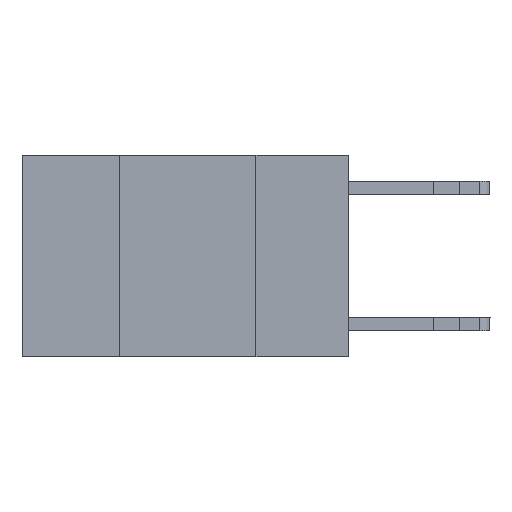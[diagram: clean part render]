
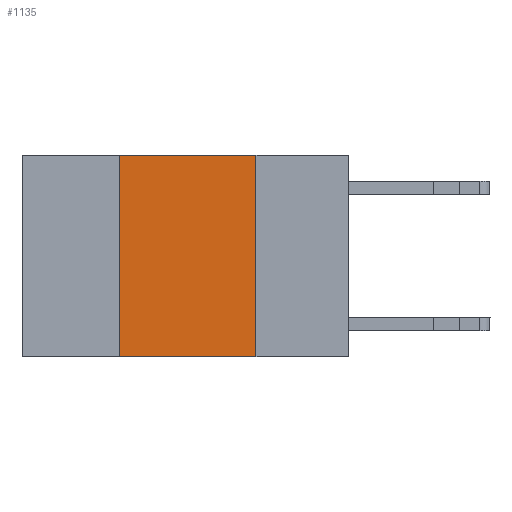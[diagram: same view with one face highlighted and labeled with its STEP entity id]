
A CAD part, left-side view. The second image highlights one B-rep face of the part: STEP entity #1135.
In plain terms, the highlighted planar face has unit normal (-1, 0, 0).
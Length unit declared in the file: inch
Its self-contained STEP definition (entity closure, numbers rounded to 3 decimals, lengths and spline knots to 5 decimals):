
#834 = DIRECTION ( 'NONE',  ( 0., 0., 1. ) ) ;
#880 = CARTESIAN_POINT ( 'NONE',  ( 0., 0.6, -0.37 ) ) ;
#1118 = CARTESIAN_POINT ( 'NONE',  ( 0., 0.17, -0.37 ) ) ;
#1135 = ADVANCED_FACE ( 'NONE', ( #6115 ), #10986, .F. ) ;
#1771 = ORIENTED_EDGE ( 'NONE', *, *, #2746, .T. ) ;
#1963 = ORIENTED_EDGE ( 'NONE', *, *, #4541, .F. ) ;
#2281 = ORIENTED_EDGE ( 'NONE', *, *, #16490, .F. ) ;
#2422 = LINE ( 'NONE', #9109, #12444 ) ;
#2746 = EDGE_CURVE ( 'NONE', #12424, #6067, #11753, .T. ) ;
#2831 = CARTESIAN_POINT ( 'NONE',  ( 0., 0.17, 0. ) ) ;
#3086 = CARTESIAN_POINT ( 'NONE',  ( 0., 0.6, 0. ) ) ;
#4416 = DIRECTION ( 'NONE',  ( 1., 0., 0. ) ) ;
#4541 = EDGE_CURVE ( 'NONE', #12424, #7056, #12873, .T. ) ;
#5389 = VECTOR ( 'NONE', #12676, 39.37008 ) ;
#5415 = EDGE_CURVE ( 'NONE', #8457, #6067, #2422, .T. ) ;
#6067 = VERTEX_POINT ( 'NONE', #1118 ) ;
#6115 = FACE_OUTER_BOUND ( 'NONE', #14345, .T. ) ;
#6760 = ORIENTED_EDGE ( 'NONE', *, *, #5415, .F. ) ;
#7056 = VERTEX_POINT ( 'NONE', #14853 ) ;
#7172 = LINE ( 'NONE', #8369, #16523 ) ;
#8369 = CARTESIAN_POINT ( 'NONE',  ( 0., 0.6, 0. ) ) ;
#8457 = VERTEX_POINT ( 'NONE', #2831 ) ;
#8743 = AXIS2_PLACEMENT_3D ( 'NONE', #3086, #4416, #13478 ) ;
#9109 = CARTESIAN_POINT ( 'NONE',  ( 0., 0.17, 0. ) ) ;
#9511 = VECTOR ( 'NONE', #834, 39.37008 ) ;
#10986 = PLANE ( 'NONE',  #8743 ) ;
#11753 = LINE ( 'NONE', #880, #5389 ) ;
#12424 = VERTEX_POINT ( 'NONE', #13159 ) ;
#12444 = VECTOR ( 'NONE', #16637, 39.37008 ) ;
#12676 = DIRECTION ( 'NONE',  ( 0., -1., 0. ) ) ;
#12873 = LINE ( 'NONE', #16338, #9511 ) ;
#13159 = CARTESIAN_POINT ( 'NONE',  ( 0., 0.42, -0.37 ) ) ;
#13478 = DIRECTION ( 'NONE',  ( 0., 0., -1. ) ) ;
#14345 = EDGE_LOOP ( 'NONE', ( #6760, #2281, #1963, #1771 ) ) ;
#14853 = CARTESIAN_POINT ( 'NONE',  ( 0., 0.42, 0. ) ) ;
#15929 = DIRECTION ( 'NONE',  ( 0., -1., 0. ) ) ;
#16338 = CARTESIAN_POINT ( 'NONE',  ( 0., 0.42, 0. ) ) ;
#16490 = EDGE_CURVE ( 'NONE', #7056, #8457, #7172, .T. ) ;
#16523 = VECTOR ( 'NONE', #15929, 39.37008 ) ;
#16637 = DIRECTION ( 'NONE',  ( 0., 0., -1. ) ) ;
